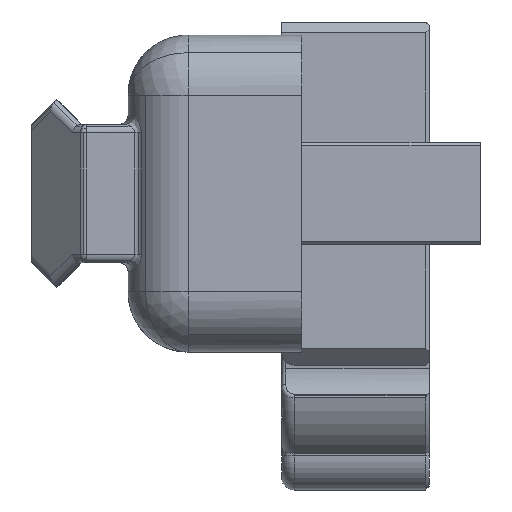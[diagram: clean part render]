
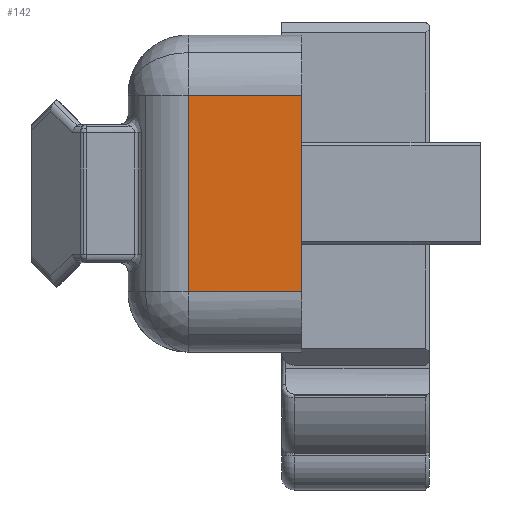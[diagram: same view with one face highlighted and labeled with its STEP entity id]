
A CAD part, front view. The second image highlights one B-rep face of the part: STEP entity #142.
In plain terms, the highlighted planar face has unit normal (0, -1, 0).
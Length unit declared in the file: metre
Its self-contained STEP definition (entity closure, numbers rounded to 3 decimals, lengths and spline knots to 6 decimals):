
#142=ADVANCED_FACE('10:25',(#536),#537,.F.);
#536=FACE_OUTER_BOUND('',#1154,.T.);
#537=PLANE('',#1155);
#1154=EDGE_LOOP('',(#2802,#2803,#2804,#2805));
#1155=AXIS2_PLACEMENT_3D('',#2806,#2807,#2808);
#2802=ORIENTED_EDGE('',*,*,#4884,.F.);
#2803=ORIENTED_EDGE('',*,*,#4879,.T.);
#2804=ORIENTED_EDGE('',*,*,#4885,.T.);
#2805=ORIENTED_EDGE('',*,*,#4875,.F.);
#2806=CARTESIAN_POINT('',(-0.203968,-0.013536,0.001));
#2807=DIRECTION('',(0.,1.0,0.));
#2808=DIRECTION('',(0.0,0.,-1.0));
#4875=EDGE_CURVE('10:673',#5948,#5950,#5951,.T.);
#4879=EDGE_CURVE('10:664',#5958,#5956,#5959,.T.);
#4884=EDGE_CURVE('10:667',#5958,#5948,#5965,.T.);
#4885=EDGE_CURVE('10:670',#5956,#5950,#5966,.F.);
#5948=VERTEX_POINT('',#7778);
#5950=VERTEX_POINT('',#7780);
#5951=LINE('',#7781,#7782);
#5956=VERTEX_POINT('',#7788);
#5958=VERTEX_POINT('',#7790);
#5959=LINE('',#7791,#7792);
#5965=LINE('',#7799,#7800);
#5966=LINE('',#7801,#7802);
#7778=CARTESIAN_POINT('',(-0.206911,-0.013536,0.012509));
#7780=CARTESIAN_POINT('',(-0.19364,-0.013536,0.012509));
#7781=CARTESIAN_POINT('',(-0.195982,-0.013536,0.012509));
#7782=VECTOR('',#9521,1.0);
#7788=CARTESIAN_POINT('',(-0.19364,-0.013536,-0.010509));
#7790=CARTESIAN_POINT('',(-0.206911,-0.013536,-0.010509));
#7791=CARTESIAN_POINT('',(-0.195982,-0.013536,-0.010509));
#7792=VECTOR('',#9529,1.0);
#7799=CARTESIAN_POINT('',(-0.206911,-0.013536,0.001));
#7800=VECTOR('',#9540,0.023019);
#7801=CARTESIAN_POINT('',(-0.19364,-0.013536,-0.01223));
#7802=VECTOR('',#9541,1.0);
#9521=DIRECTION('',(1.0,0.,0.));
#9529=DIRECTION('',(1.0,0.,0.));
#9540=DIRECTION('',(0.,0.,1.0));
#9541=DIRECTION('',(0.,0.,-1.));
